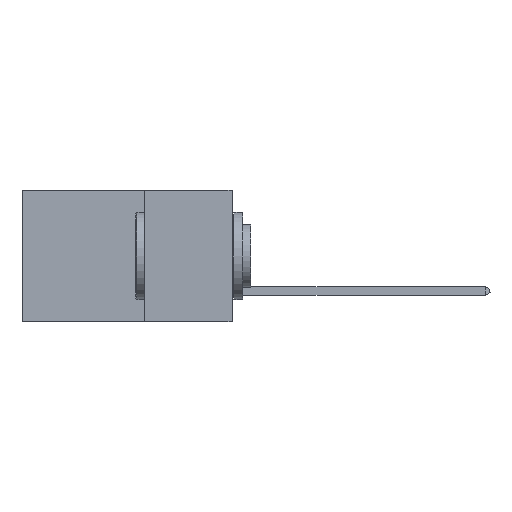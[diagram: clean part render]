
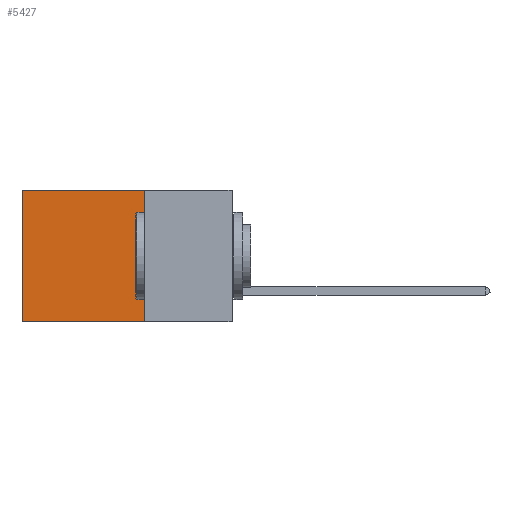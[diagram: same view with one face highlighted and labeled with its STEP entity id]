
A CAD part, left-side view. The second image highlights one B-rep face of the part: STEP entity #5427.
In plain terms, the highlighted planar face has unit normal (-1, 0, 0).
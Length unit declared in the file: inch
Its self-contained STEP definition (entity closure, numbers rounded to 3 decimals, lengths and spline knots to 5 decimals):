
#489 = CARTESIAN_POINT ( 'NONE',  ( 0.2875, 0.6, -0.375 ) ) ;
#561 = ORIENTED_EDGE ( 'NONE', *, *, #7757, .F. ) ;
#898 = LINE ( 'NONE', #13567, #6055 ) ;
#1147 = CARTESIAN_POINT ( 'NONE',  ( 0.2875, 0.25, -0.375 ) ) ;
#2844 = CARTESIAN_POINT ( 'NONE',  ( 0.2875, 0.6, -0.375 ) ) ;
#3065 = CARTESIAN_POINT ( 'NONE',  ( 0.2875, 0.25, -0.375 ) ) ;
#3423 = LINE ( 'NONE', #2844, #9891 ) ;
#3729 = LINE ( 'NONE', #13108, #10576 ) ;
#4245 = VERTEX_POINT ( 'NONE', #11810 ) ;
#4439 = CARTESIAN_POINT ( 'NONE',  ( 0.2875, 0.25, -0.375 ) ) ;
#4999 = ORIENTED_EDGE ( 'NONE', *, *, #15385, .T. ) ;
#5142 = DIRECTION ( 'NONE',  ( 0., 0., -1. ) ) ;
#5427 = ADVANCED_FACE ( 'NONE', ( #6058 ), #9134, .F. ) ;
#5799 = LINE ( 'NONE', #4439, #13557 ) ;
#6055 = VECTOR ( 'NONE', #11176, 39.37008 ) ;
#6058 = FACE_OUTER_BOUND ( 'NONE', #13558, .T. ) ;
#7757 = EDGE_CURVE ( 'NONE', #8464, #12666, #898, .T. ) ;
#7916 = DIRECTION ( 'NONE',  ( 0., 0., -1. ) ) ;
#8464 = VERTEX_POINT ( 'NONE', #14815 ) ;
#9134 = PLANE ( 'NONE',  #11544 ) ;
#9891 = VECTOR ( 'NONE', #5142, 39.37008 ) ;
#10576 = VECTOR ( 'NONE', #15393, 39.37008 ) ;
#11176 = DIRECTION ( 'NONE',  ( 0., 0., -1. ) ) ;
#11544 = AXIS2_PLACEMENT_3D ( 'NONE', #3065, #15171, #7916 ) ;
#11627 = VERTEX_POINT ( 'NONE', #489 ) ;
#11640 = DIRECTION ( 'NONE',  ( 0., 1., 0. ) ) ;
#11810 = CARTESIAN_POINT ( 'NONE',  ( 0.2875, 0.6, 0. ) ) ;
#11979 = ORIENTED_EDGE ( 'NONE', *, *, #12613, .T. ) ;
#12613 = EDGE_CURVE ( 'NONE', #8464, #4245, #3729, .T. ) ;
#12666 = VERTEX_POINT ( 'NONE', #1147 ) ;
#12669 = ORIENTED_EDGE ( 'NONE', *, *, #13644, .F. ) ;
#13108 = CARTESIAN_POINT ( 'NONE',  ( 0.2875, 0.25, 0. ) ) ;
#13557 = VECTOR ( 'NONE', #11640, 39.37008 ) ;
#13558 = EDGE_LOOP ( 'NONE', ( #4999, #12669, #561, #11979 ) ) ;
#13567 = CARTESIAN_POINT ( 'NONE',  ( 0.2875, 0.25, -0.375 ) ) ;
#13644 = EDGE_CURVE ( 'NONE', #12666, #11627, #5799, .T. ) ;
#14815 = CARTESIAN_POINT ( 'NONE',  ( 0.2875, 0.25, 0. ) ) ;
#15171 = DIRECTION ( 'NONE',  ( 1., 0., 0. ) ) ;
#15385 = EDGE_CURVE ( 'NONE', #4245, #11627, #3423, .T. ) ;
#15393 = DIRECTION ( 'NONE',  ( 0., 1., 0. ) ) ;
